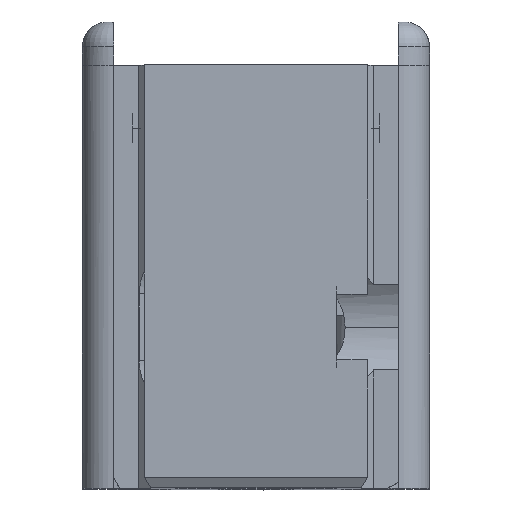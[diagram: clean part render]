
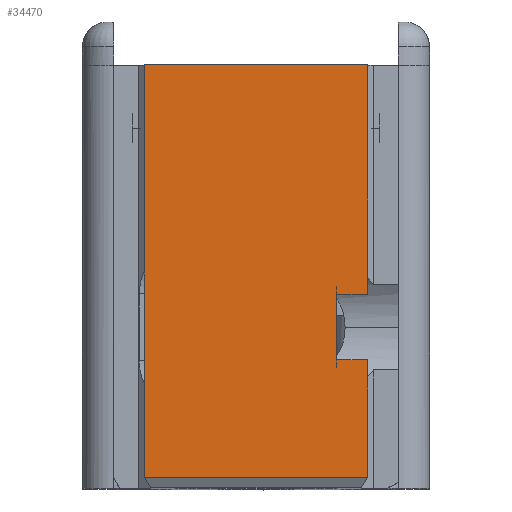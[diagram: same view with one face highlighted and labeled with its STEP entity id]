
A CAD part, top view. The second image highlights one B-rep face of the part: STEP entity #34470.
In plain terms, the highlighted planar face has unit normal (0, 0, 1).
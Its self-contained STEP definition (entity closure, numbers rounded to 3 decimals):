
#500 = LINE ( 'NONE', #18873, #53620 ) ;
#4982 = EDGE_CURVE ( 'NONE', #7910, #22218, #24176, .T. ) ;
#5453 = CARTESIAN_POINT ( 'NONE',  ( 9., 14.641, 34.7 ) ) ;
#5994 = ORIENTED_EDGE ( 'NONE', *, *, #45689, .T. ) ;
#7527 = CARTESIAN_POINT ( 'NONE',  ( 6.5, 33.15, 34.7 ) ) ;
#7910 = VERTEX_POINT ( 'NONE', #38539 ) ;
#8200 = DIRECTION ( 'NONE',  ( 1., 0., 0. ) ) ;
#8695 = LINE ( 'NONE', #31337, #56726 ) ;
#8732 = DIRECTION ( 'NONE',  ( 0., 1., 0. ) ) ;
#12725 = ORIENTED_EDGE ( 'NONE', *, *, #14585, .F. ) ;
#13267 = DIRECTION ( 'NONE',  ( 0., -1., 0. ) ) ;
#14036 = DIRECTION ( 'NONE',  ( 0., 0., 1. ) ) ;
#14585 = EDGE_CURVE ( 'NONE', #33922, #22957, #8695, .T. ) ;
#14612 = AXIS2_PLACEMENT_3D ( 'NONE', #36769, #14036, #41474 ) ;
#17741 = DIRECTION ( 'NONE',  ( 0., -1., 0. ) ) ;
#18873 = CARTESIAN_POINT ( 'NONE',  ( 9., -0.134, 34.7 ) ) ;
#22218 = VERTEX_POINT ( 'NONE', #5453 ) ;
#22365 = VECTOR ( 'NONE', #44714, 1000. ) ;
#22383 = CARTESIAN_POINT ( 'NONE',  ( -9., 33.15, 34.7 ) ) ;
#22604 = EDGE_LOOP ( 'NONE', ( #5994, #53084, #52735, #12725, #33519, #46151, #33767, #36434 ) ) ;
#22908 = VERTEX_POINT ( 'NONE', #45750 ) ;
#22957 = VERTEX_POINT ( 'NONE', #37189 ) ;
#23833 = LINE ( 'NONE', #60388, #22365 ) ;
#24176 = LINE ( 'NONE', #35839, #49642 ) ;
#26363 = CARTESIAN_POINT ( 'NONE',  ( -9., -0.134, 34.7 ) ) ;
#27452 = LINE ( 'NONE', #7527, #58777 ) ;
#28587 = VECTOR ( 'NONE', #56199, 1000. ) ;
#28636 = FACE_OUTER_BOUND ( 'NONE', #22604, .T. ) ;
#30387 = LINE ( 'NONE', #41316, #39845 ) ;
#31337 = CARTESIAN_POINT ( 'NONE',  ( 6.5, 9.329, 34.7 ) ) ;
#33106 = DIRECTION ( 'NONE',  ( 1., 0., 0. ) ) ;
#33519 = ORIENTED_EDGE ( 'NONE', *, *, #44692, .T. ) ;
#33767 = ORIENTED_EDGE ( 'NONE', *, *, #4982, .F. ) ;
#33922 = VERTEX_POINT ( 'NONE', #54797 ) ;
#34361 = CARTESIAN_POINT ( 'NONE',  ( 6.5, 14.641, 34.7 ) ) ;
#34470 = ADVANCED_FACE ( 'NONE', ( #28636 ), #41893, .T. ) ;
#35839 = CARTESIAN_POINT ( 'NONE',  ( 9., 33.15, 34.7 ) ) ;
#36189 = EDGE_CURVE ( 'NONE', #56996, #7910, #54118, .T. ) ;
#36434 = ORIENTED_EDGE ( 'NONE', *, *, #36189, .F. ) ;
#36769 = CARTESIAN_POINT ( 'NONE',  ( -9., 33.15, 34.7 ) ) ;
#37189 = CARTESIAN_POINT ( 'NONE',  ( 9., 9.329, 34.7 ) ) ;
#37842 = VECTOR ( 'NONE', #52239, 1000. ) ;
#38539 = CARTESIAN_POINT ( 'NONE',  ( 9., 33.15, 34.7 ) ) ;
#39845 = VECTOR ( 'NONE', #13267, 1000. ) ;
#41316 = CARTESIAN_POINT ( 'NONE',  ( -9., 33.15, 34.7 ) ) ;
#41474 = DIRECTION ( 'NONE',  ( 1., 0., 0. ) ) ;
#41490 = LINE ( 'NONE', #53028, #37842 ) ;
#41893 = PLANE ( 'NONE',  #14612 ) ;
#44692 = EDGE_CURVE ( 'NONE', #33922, #46029, #27452, .T. ) ;
#44702 = EDGE_CURVE ( 'NONE', #22957, #22908, #23833, .T. ) ;
#44714 = DIRECTION ( 'NONE',  ( 0., -1., 0. ) ) ;
#44759 = EDGE_CURVE ( 'NONE', #54028, #22908, #500, .T. ) ;
#45689 = EDGE_CURVE ( 'NONE', #56996, #54028, #30387, .T. ) ;
#45750 = CARTESIAN_POINT ( 'NONE',  ( 9., -0.134, 34.7 ) ) ;
#46029 = VERTEX_POINT ( 'NONE', #34361 ) ;
#46151 = ORIENTED_EDGE ( 'NONE', *, *, #52105, .F. ) ;
#47618 = CARTESIAN_POINT ( 'NONE',  ( -9., 33.15, 34.7 ) ) ;
#49642 = VECTOR ( 'NONE', #17741, 1000. ) ;
#52105 = EDGE_CURVE ( 'NONE', #22218, #46029, #41490, .T. ) ;
#52239 = DIRECTION ( 'NONE',  ( -1., 0., 0. ) ) ;
#52735 = ORIENTED_EDGE ( 'NONE', *, *, #44702, .F. ) ;
#53028 = CARTESIAN_POINT ( 'NONE',  ( 6.5, 14.641, 34.7 ) ) ;
#53084 = ORIENTED_EDGE ( 'NONE', *, *, #44759, .T. ) ;
#53620 = VECTOR ( 'NONE', #33106, 1000. ) ;
#54028 = VERTEX_POINT ( 'NONE', #26363 ) ;
#54118 = LINE ( 'NONE', #47618, #28587 ) ;
#54797 = CARTESIAN_POINT ( 'NONE',  ( 6.5, 9.329, 34.7 ) ) ;
#56199 = DIRECTION ( 'NONE',  ( 1., 0., 0. ) ) ;
#56726 = VECTOR ( 'NONE', #8200, 1000. ) ;
#56996 = VERTEX_POINT ( 'NONE', #22383 ) ;
#58777 = VECTOR ( 'NONE', #8732, 1000. ) ;
#60388 = CARTESIAN_POINT ( 'NONE',  ( 9., 33.15, 34.7 ) ) ;
